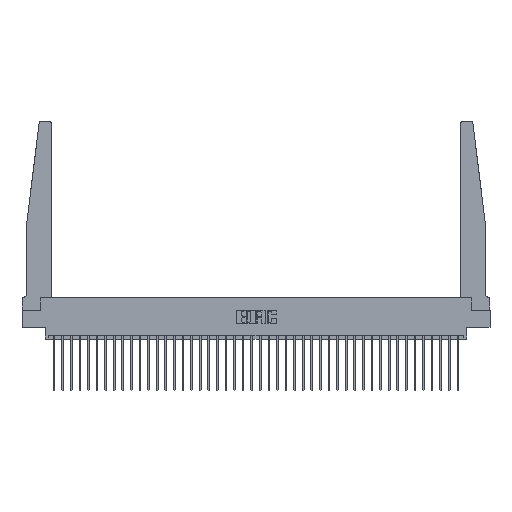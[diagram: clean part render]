
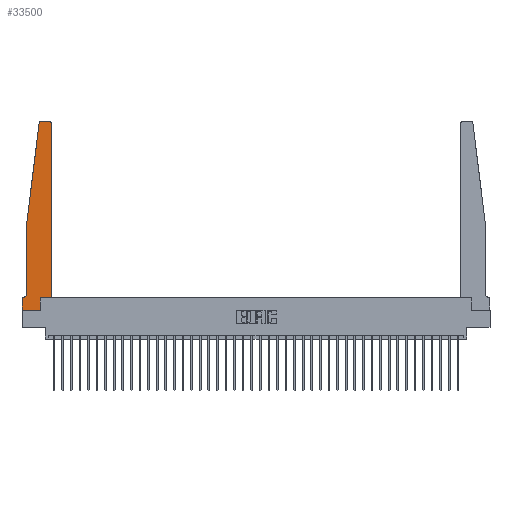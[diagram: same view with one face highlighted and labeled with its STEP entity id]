
A CAD part, top view. The second image highlights one B-rep face of the part: STEP entity #33500.
In plain terms, the highlighted planar face has unit normal (0, 0, 1).
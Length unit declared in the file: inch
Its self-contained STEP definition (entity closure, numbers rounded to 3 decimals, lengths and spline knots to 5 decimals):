
#75 = EDGE_CURVE ( 'NONE', #34825, #5789, #22224, .T. ) ;
#500 = DIRECTION ( 'NONE',  ( 0., -1., 0. ) ) ;
#2170 = ORIENTED_EDGE ( 'NONE', *, *, #6807, .T. ) ;
#3292 = VERTEX_POINT ( 'NONE', #32447 ) ;
#3444 = CARTESIAN_POINT ( 'NONE',  ( 0.015, 0.1875, 0.37 ) ) ;
#3600 = CARTESIAN_POINT ( 'NONE',  ( 0.2605, 0., 0.37 ) ) ;
#4679 = EDGE_CURVE ( 'NONE', #10124, #25960, #28520, .T. ) ;
#5112 = ORIENTED_EDGE ( 'NONE', *, *, #75, .T. ) ;
#5129 = LINE ( 'NONE', #29653, #18760 ) ;
#5461 = EDGE_CURVE ( 'NONE', #26974, #10124, #6250, .T. ) ;
#5789 = VERTEX_POINT ( 'NONE', #27590 ) ;
#5967 = LINE ( 'NONE', #19567, #27764 ) ;
#5984 = DIRECTION ( 'NONE',  ( -1., 0., 0. ) ) ;
#6250 = LINE ( 'NONE', #20679, #26314 ) ;
#6340 = CIRCLE ( 'NONE', #20268, 0.03 ) ;
#6807 = EDGE_CURVE ( 'NONE', #13342, #34825, #30133, .T. ) ;
#7710 = VECTOR ( 'NONE', #21315, 39.37008 ) ;
#8746 = CARTESIAN_POINT ( 'NONE',  ( 0.395, 2.72, 0.37 ) ) ;
#8850 = DIRECTION ( 'NONE',  ( 0., 0., 1. ) ) ;
#9286 = EDGE_CURVE ( 'NONE', #5789, #26974, #13671, .T. ) ;
#9832 = DIRECTION ( 'NONE',  ( 1., 0., 0. ) ) ;
#10034 = EDGE_CURVE ( 'NONE', #34161, #17497, #5967, .T. ) ;
#10124 = VERTEX_POINT ( 'NONE', #3600 ) ;
#10518 = CARTESIAN_POINT ( 'NONE',  ( 0.27653, 2.75, 0.37 ) ) ;
#10788 = ORIENTED_EDGE ( 'NONE', *, *, #23259, .T. ) ;
#11448 = DIRECTION ( 'NONE',  ( 1., 0., 0. ) ) ;
#11477 = ORIENTED_EDGE ( 'NONE', *, *, #17726, .T. ) ;
#11517 = CARTESIAN_POINT ( 'NONE',  ( 0.2605, 0.18, 0.37 ) ) ;
#11532 = VERTEX_POINT ( 'NONE', #31745 ) ;
#12013 = LINE ( 'NONE', #19492, #31273 ) ;
#12683 = DIRECTION ( 'NONE',  ( 0., 0., -1. ) ) ;
#13342 = VERTEX_POINT ( 'NONE', #17493 ) ;
#13391 = ORIENTED_EDGE ( 'NONE', *, *, #35000, .T. ) ;
#13671 = LINE ( 'NONE', #22148, #20099 ) ;
#14298 = VECTOR ( 'NONE', #31415, 39.37008 ) ;
#15234 = CARTESIAN_POINT ( 'NONE',  ( 0.395, 2.75, 0.37 ) ) ;
#15513 = DIRECTION ( 'NONE',  ( 0., 0., 1. ) ) ;
#17238 = ORIENTED_EDGE ( 'NONE', *, *, #4679, .T. ) ;
#17279 = CARTESIAN_POINT ( 'NONE',  ( 0.2605, 0.18, 0.37 ) ) ;
#17493 = CARTESIAN_POINT ( 'NONE',  ( 0.065, 0.2375, 0.37 ) ) ;
#17497 = VERTEX_POINT ( 'NONE', #10518 ) ;
#17726 = EDGE_CURVE ( 'NONE', #3292, #34161, #6340, .T. ) ;
#18760 = VECTOR ( 'NONE', #32420, 39.37008 ) ;
#19492 = CARTESIAN_POINT ( 'NONE',  ( 0.065, 1.25, 0.37 ) ) ;
#19567 = CARTESIAN_POINT ( 'NONE',  ( 0.25, 2.75, 0.37 ) ) ;
#20099 = VECTOR ( 'NONE', #33164, 39.37008 ) ;
#20268 = AXIS2_PLACEMENT_3D ( 'NONE', #8746, #27826, #11448 ) ;
#20679 = CARTESIAN_POINT ( 'NONE',  ( 0., 0., 0.37 ) ) ;
#21210 = AXIS2_PLACEMENT_3D ( 'NONE', #29085, #12683, #31840 ) ;
#21315 = DIRECTION ( 'NONE',  ( -1., 0., 0. ) ) ;
#21757 = CARTESIAN_POINT ( 'NONE',  ( 0., 0., 0.37 ) ) ;
#21907 = AXIS2_PLACEMENT_3D ( 'NONE', #31934, #15513, #34700 ) ;
#22148 = CARTESIAN_POINT ( 'NONE',  ( 0., 0., 0.37 ) ) ;
#22224 = LINE ( 'NONE', #26826, #7710 ) ;
#22269 = CARTESIAN_POINT ( 'NONE',  ( 0.425, 0.18, 0.37 ) ) ;
#22459 = LINE ( 'NONE', #23141, #14298 ) ;
#22801 = ORIENTED_EDGE ( 'NONE', *, *, #9286, .T. ) ;
#23141 = CARTESIAN_POINT ( 'NONE',  ( 0.065, 1.25, 0.37 ) ) ;
#23259 = EDGE_CURVE ( 'NONE', #31358, #3292, #5129, .T. ) ;
#23574 = VERTEX_POINT ( 'NONE', #28333 ) ;
#23659 = PLANE ( 'NONE',  #21907 ) ;
#24236 = FACE_OUTER_BOUND ( 'NONE', #24837, .T. ) ;
#24709 = ORIENTED_EDGE ( 'NONE', *, *, #31326, .T. ) ;
#24837 = EDGE_LOOP ( 'NONE', ( #30476, #27451, #13391, #24709, #2170, #5112, #22801, #33032, #17238, #30254, #10788, #11477 ) ) ;
#25155 = CARTESIAN_POINT ( 'NONE',  ( 0.27653, 2.72, 0.37 ) ) ;
#25251 = CARTESIAN_POINT ( 'NONE',  ( 0.425, 0.18, 0.37 ) ) ;
#25468 = AXIS2_PLACEMENT_3D ( 'NONE', #25155, #8850, #27940 ) ;
#25960 = VERTEX_POINT ( 'NONE', #17279 ) ;
#26314 = VECTOR ( 'NONE', #9832, 39.37008 ) ;
#26826 = CARTESIAN_POINT ( 'NONE',  ( 0.065, 0.1875, 0.37 ) ) ;
#26974 = VERTEX_POINT ( 'NONE', #21757 ) ;
#27451 = ORIENTED_EDGE ( 'NONE', *, *, #28771, .T. ) ;
#27590 = CARTESIAN_POINT ( 'NONE',  ( 0., 0.1875, 0.37 ) ) ;
#27764 = VECTOR ( 'NONE', #5984, 39.37008 ) ;
#27826 = DIRECTION ( 'NONE',  ( 0., 0., 1. ) ) ;
#27908 = DIRECTION ( 'NONE',  ( 0., 1., 0. ) ) ;
#27940 = DIRECTION ( 'NONE',  ( 1., 0., 0. ) ) ;
#28333 = CARTESIAN_POINT ( 'NONE',  ( 0.24675, 2.72367, 0.37 ) ) ;
#28520 = LINE ( 'NONE', #11517, #34941 ) ;
#28771 = EDGE_CURVE ( 'NONE', #17497, #23574, #35042, .T. ) ;
#29085 = CARTESIAN_POINT ( 'NONE',  ( 0.015, 0.2375, 0.37 ) ) ;
#29653 = CARTESIAN_POINT ( 'NONE',  ( 0.425, 0.18, 0.37 ) ) ;
#29835 = LINE ( 'NONE', #22269, #35436 ) ;
#30133 = CIRCLE ( 'NONE', #21210, 0.05 ) ;
#30254 = ORIENTED_EDGE ( 'NONE', *, *, #33125, .T. ) ;
#30476 = ORIENTED_EDGE ( 'NONE', *, *, #10034, .T. ) ;
#31273 = VECTOR ( 'NONE', #500, 39.37008 ) ;
#31326 = EDGE_CURVE ( 'NONE', #11532, #13342, #12013, .T. ) ;
#31358 = VERTEX_POINT ( 'NONE', #25251 ) ;
#31415 = DIRECTION ( 'NONE',  ( -0.122, -0.992, 0. ) ) ;
#31745 = CARTESIAN_POINT ( 'NONE',  ( 0.065, 1.25, 0.37 ) ) ;
#31840 = DIRECTION ( 'NONE',  ( -1., 0., 0. ) ) ;
#31934 = CARTESIAN_POINT ( 'NONE',  ( 0., 0.1875, 0.37 ) ) ;
#32420 = DIRECTION ( 'NONE',  ( 0., 1., 0. ) ) ;
#32447 = CARTESIAN_POINT ( 'NONE',  ( 0.425, 2.72, 0.37 ) ) ;
#33032 = ORIENTED_EDGE ( 'NONE', *, *, #5461, .T. ) ;
#33125 = EDGE_CURVE ( 'NONE', #25960, #31358, #29835, .T. ) ;
#33157 = DIRECTION ( 'NONE',  ( 1., 0., 0. ) ) ;
#33164 = DIRECTION ( 'NONE',  ( 0., -1., 0. ) ) ;
#33500 = ADVANCED_FACE ( 'NONE', ( #24236 ), #23659, .T. ) ;
#34161 = VERTEX_POINT ( 'NONE', #15234 ) ;
#34700 = DIRECTION ( 'NONE',  ( 1., 0., 0. ) ) ;
#34825 = VERTEX_POINT ( 'NONE', #3444 ) ;
#34941 = VECTOR ( 'NONE', #27908, 39.37008 ) ;
#35000 = EDGE_CURVE ( 'NONE', #23574, #11532, #22459, .T. ) ;
#35042 = CIRCLE ( 'NONE', #25468, 0.03 ) ;
#35436 = VECTOR ( 'NONE', #33157, 39.37008 ) ;
